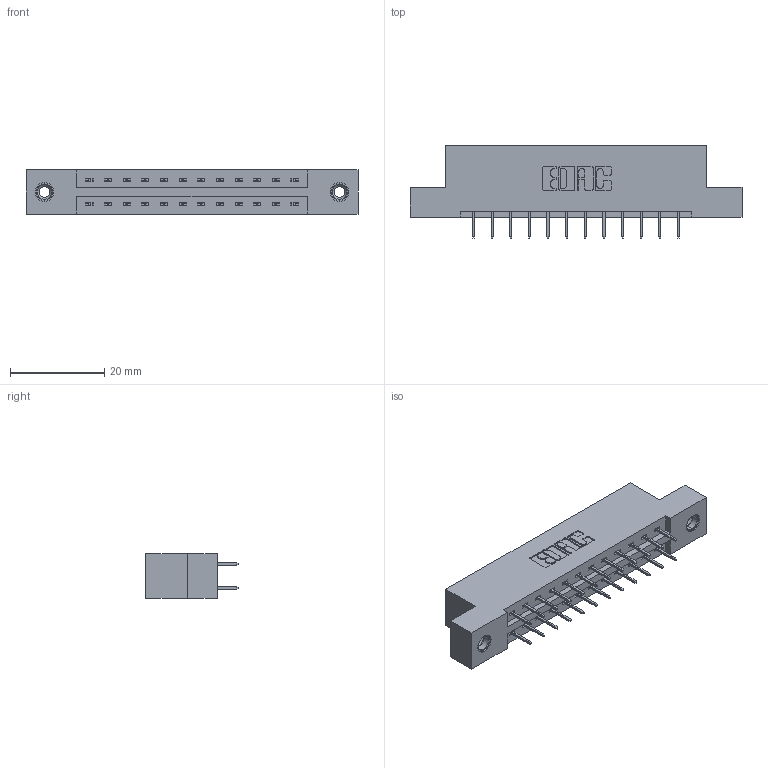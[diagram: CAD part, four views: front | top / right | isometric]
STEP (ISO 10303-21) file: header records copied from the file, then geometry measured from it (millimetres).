
FILE_DESCRIPTION (( 'STEP AP203' ), '1' );
FILE_NAME ('387-024-524-208.STEP', '2019-10-16T18:04:11', ( '' ), ( '' ), 'SwSTEP 2.0', 'SolidWorks 2016', '' );
FILE_SCHEMA (( 'CONFIG_CONTROL_DESIGN' ));
Length unit declared in the file: inch
Products named in the file (4): 345-250-001_345-250-003-102; 387-024-524-208; 337 Part_Flush Mounting Lugs - 0.156 Dia-TI; 345-292-001_345-293-124
Assembly tree (27 placements, depth 2):
  387-024-524-208
    337 Part_Flush Mounting Lugs - 0.156 Dia-TI
    345-292-001_345-293-124  x24
    345-250-001_345-250-003-102  x2
Bounding box: 70.56 x 19.69 x 9.4 mm (x, y, z)
Volume: 6994.1 mm3; surface area: 7526.9 mm2
Topology: 27 solids, 27 shells, 1566 faces, 4407 edges, 2834 vertices
Faces by surface type: plane 1158, cylinder 392, cone 12, torus 4
Entity records: 14444 total; most frequent: CARTESIAN_POINT 2437, ORIENTED_EDGE 2366, DIRECTION 2161, EDGE_CURVE 1183, LINE 1039, VECTOR 1039, VERTEX_POINT 780, AXIS2_PLACEMENT_3D 561
